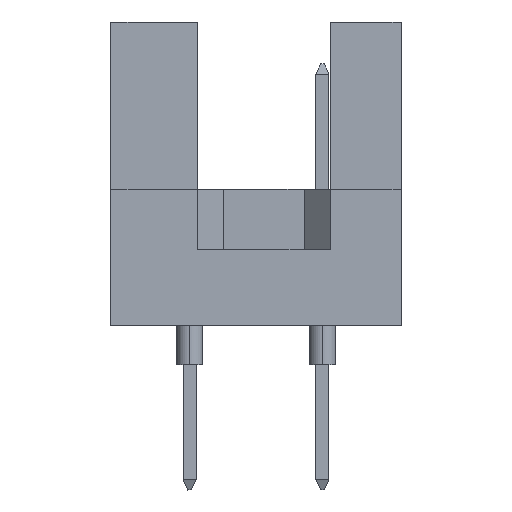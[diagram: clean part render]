
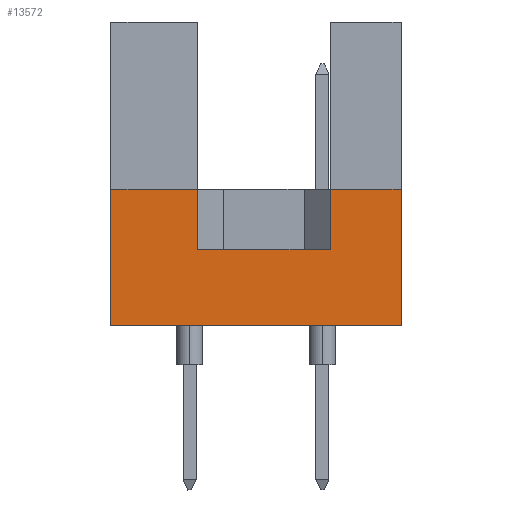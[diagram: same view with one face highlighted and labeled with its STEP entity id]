
A CAD part, left-side view. The second image highlights one B-rep face of the part: STEP entity #13572.
In plain terms, the highlighted planar face has unit normal (-1, 0, 0).
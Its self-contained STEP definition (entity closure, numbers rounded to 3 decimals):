
#196 = EDGE_CURVE ( 'NONE', #4887, #3514, #16020, .T. ) ;
#537 = EDGE_CURVE ( 'NONE', #9908, #3942, #11701, .T. ) ;
#733 = CARTESIAN_POINT ( 'NONE',  ( -47.5, 0., 0. ) ) ;
#967 = CARTESIAN_POINT ( 'NONE',  ( -47.5, 11.1, 0. ) ) ;
#2232 = VERTEX_POINT ( 'NONE', #9141 ) ;
#2347 = FACE_OUTER_BOUND ( 'NONE', #16323, .T. ) ;
#3024 = VECTOR ( 'NONE', #11937, 1000. ) ;
#3136 = DIRECTION ( 'NONE',  ( 0., 0., -1. ) ) ;
#3514 = VERTEX_POINT ( 'NONE', #16962 ) ;
#3687 = VECTOR ( 'NONE', #10556, 1000. ) ;
#3790 = DIRECTION ( 'NONE',  ( 0., -1., 0. ) ) ;
#3911 = EDGE_CURVE ( 'NONE', #4923, #4887, #15504, .T. ) ;
#3913 = ORIENTED_EDGE ( 'NONE', *, *, #537, .F. ) ;
#3942 = VERTEX_POINT ( 'NONE', #6029 ) ;
#4405 = ORIENTED_EDGE ( 'NONE', *, *, #11452, .T. ) ;
#4887 = VERTEX_POINT ( 'NONE', #14271 ) ;
#4923 = VERTEX_POINT ( 'NONE', #967 ) ;
#5077 = ORIENTED_EDGE ( 'NONE', *, *, #9685, .T. ) ;
#5156 = LINE ( 'NONE', #9597, #3024 ) ;
#5482 = ORIENTED_EDGE ( 'NONE', *, *, #3911, .F. ) ;
#6015 = LINE ( 'NONE', #8955, #12186 ) ;
#6029 = CARTESIAN_POINT ( 'NONE',  ( -47.5, 0., 5.2 ) ) ;
#6189 = VECTOR ( 'NONE', #7069, 1000. ) ;
#6312 = ORIENTED_EDGE ( 'NONE', *, *, #7192, .F. ) ;
#6949 = PLANE ( 'NONE',  #12648 ) ;
#7057 = CARTESIAN_POINT ( 'NONE',  ( -47.5, 2.71, 2.9 ) ) ;
#7069 = DIRECTION ( 'NONE',  ( 0., 0., 1. ) ) ;
#7192 = EDGE_CURVE ( 'NONE', #15714, #9509, #5156, .T. ) ;
#7364 = DIRECTION ( 'NONE',  ( 0., 0., 1. ) ) ;
#7680 = LINE ( 'NONE', #733, #14157 ) ;
#7784 = VECTOR ( 'NONE', #7364, 1000. ) ;
#8868 = DIRECTION ( 'NONE',  ( 0., -1., 0. ) ) ;
#8955 = CARTESIAN_POINT ( 'NONE',  ( -47.5, 11.1, 0. ) ) ;
#8995 = ORIENTED_EDGE ( 'NONE', *, *, #13070, .T. ) ;
#9141 = CARTESIAN_POINT ( 'NONE',  ( -47.5, 0., 0. ) ) ;
#9509 = VERTEX_POINT ( 'NONE', #7057 ) ;
#9597 = CARTESIAN_POINT ( 'NONE',  ( -47.5, 7.79, 2.9 ) ) ;
#9666 = VECTOR ( 'NONE', #3790, 1000. ) ;
#9685 = EDGE_CURVE ( 'NONE', #2232, #3942, #7680, .T. ) ;
#9897 = CARTESIAN_POINT ( 'NONE',  ( -47.5, 11.1, 0. ) ) ;
#9908 = VERTEX_POINT ( 'NONE', #16089 ) ;
#9956 = VECTOR ( 'NONE', #14217, 1000. ) ;
#10085 = DIRECTION ( 'NONE',  ( 0., 0., 1. ) ) ;
#10556 = DIRECTION ( 'NONE',  ( 0., 0., 1. ) ) ;
#10909 = LINE ( 'NONE', #12603, #6189 ) ;
#11452 = EDGE_CURVE ( 'NONE', #4923, #2232, #6015, .T. ) ;
#11701 = LINE ( 'NONE', #17174, #9956 ) ;
#11937 = DIRECTION ( 'NONE',  ( 0., -1., 0. ) ) ;
#12158 = LINE ( 'NONE', #17374, #3687 ) ;
#12186 = VECTOR ( 'NONE', #8868, 1000. ) ;
#12603 = CARTESIAN_POINT ( 'NONE',  ( -47.5, 2.71, 2.9 ) ) ;
#12648 = AXIS2_PLACEMENT_3D ( 'NONE', #9897, #13741, #3136 ) ;
#12809 = CARTESIAN_POINT ( 'NONE',  ( -47.5, 11.1, 0. ) ) ;
#13070 = EDGE_CURVE ( 'NONE', #15714, #3514, #12158, .T. ) ;
#13572 = ADVANCED_FACE ( 'NONE', ( #2347 ), #6949, .F. ) ;
#13741 = DIRECTION ( 'NONE',  ( 1., 0., 0. ) ) ;
#14157 = VECTOR ( 'NONE', #10085, 1000. ) ;
#14217 = DIRECTION ( 'NONE',  ( 0., -1., 0. ) ) ;
#14271 = CARTESIAN_POINT ( 'NONE',  ( -47.5, 11.1, 5.2 ) ) ;
#15504 = LINE ( 'NONE', #12809, #7784 ) ;
#15714 = VERTEX_POINT ( 'NONE', #17482 ) ;
#15873 = ORIENTED_EDGE ( 'NONE', *, *, #196, .F. ) ;
#16020 = LINE ( 'NONE', #16202, #9666 ) ;
#16089 = CARTESIAN_POINT ( 'NONE',  ( -47.5, 2.71, 5.2 ) ) ;
#16184 = ORIENTED_EDGE ( 'NONE', *, *, #17599, .F. ) ;
#16202 = CARTESIAN_POINT ( 'NONE',  ( -47.5, 11.1, 5.2 ) ) ;
#16323 = EDGE_LOOP ( 'NONE', ( #6312, #8995, #15873, #5482, #4405, #5077, #3913, #16184 ) ) ;
#16962 = CARTESIAN_POINT ( 'NONE',  ( -47.5, 7.79, 5.2 ) ) ;
#17174 = CARTESIAN_POINT ( 'NONE',  ( -47.5, 11.1, 5.2 ) ) ;
#17374 = CARTESIAN_POINT ( 'NONE',  ( -47.5, 7.79, 2.9 ) ) ;
#17482 = CARTESIAN_POINT ( 'NONE',  ( -47.5, 7.79, 2.9 ) ) ;
#17599 = EDGE_CURVE ( 'NONE', #9509, #9908, #10909, .T. ) ;
